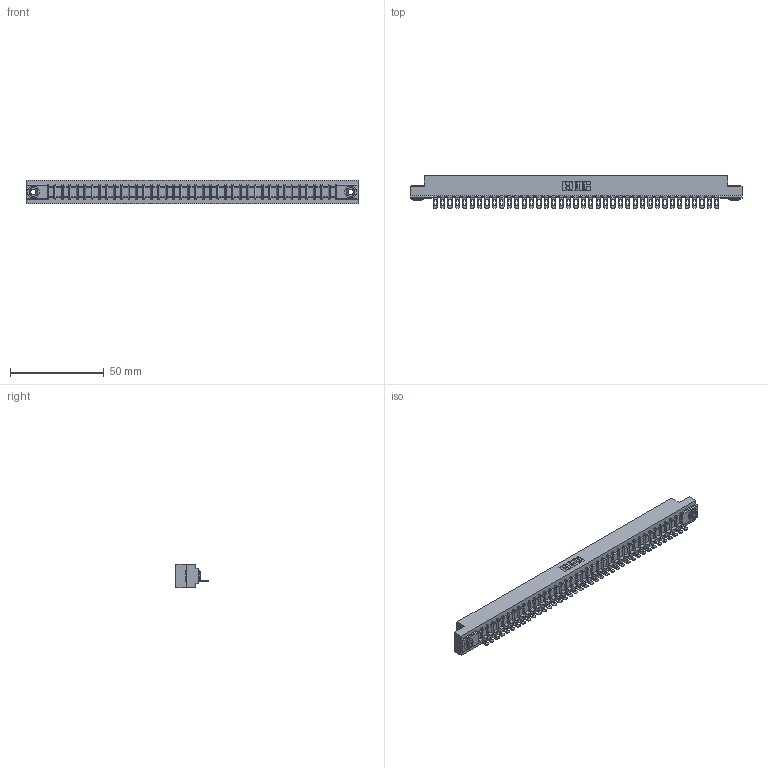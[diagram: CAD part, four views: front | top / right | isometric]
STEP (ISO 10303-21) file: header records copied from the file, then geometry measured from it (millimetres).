
FILE_DESCRIPTION (( 'STEP AP203' ), '1' );
FILE_NAME ('307-039-501-103.STEP', '2018-08-05T12:54:24', ( '' ), ( '' ), 'SwSTEP 2.0', 'SolidWorks 2016', '' );
FILE_SCHEMA (( 'CONFIG_CONTROL_DESIGN' ));
Length unit declared in the file: inch
Products named in the file (4): 307-039-501-103; 307 Part_.156 Dia Mounting Holes; 307-290-002_501; 345-250-002_345-250-002-102
Assembly tree (42 placements, depth 2):
  307-039-501-103
    307 Part_.156 Dia Mounting Holes
    307-290-002_501  x39
    345-250-002_345-250-002-102  x2
Bounding box: 177.55 x 17.42 x 12.7 mm (x, y, z)
Volume: 19012.6 mm3; surface area: 24352.5 mm2
Topology: 42 solids, 42 shells, 3174 faces, 9717 edges, 6366 vertices
Faces by surface type: plane 1810, cylinder 1276, sphere 80, cone 8
Entity records: 35663 total; most frequent: CARTESIAN_POINT 5993, ORIENTED_EDGE 5974, DIRECTION 5843, EDGE_CURVE 2987, LINE 2275, VECTOR 2275, VERTEX_POINT 1934, AXIS2_PLACEMENT_3D 1784
